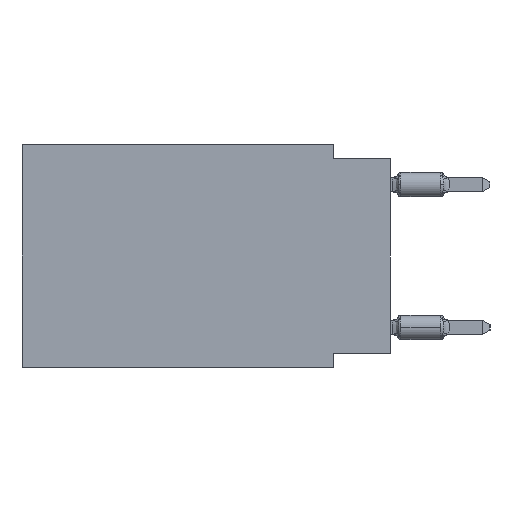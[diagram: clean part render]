
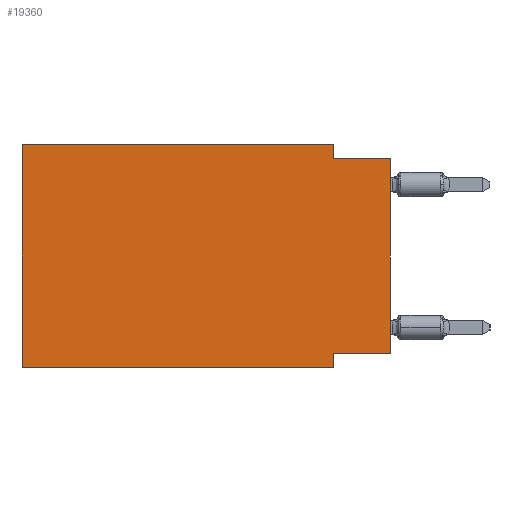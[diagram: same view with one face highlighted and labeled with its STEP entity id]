
A CAD part, left-side view. The second image highlights one B-rep face of the part: STEP entity #19360.
In plain terms, the highlighted planar face has unit normal (-1, 0, 0).
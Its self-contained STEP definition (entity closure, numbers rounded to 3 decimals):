
#542 = VERTEX_POINT ( 'NONE', #7815 ) ;
#738 = FACE_OUTER_BOUND ( 'NONE', #15789, .T. ) ;
#1135 = CARTESIAN_POINT ( 'NONE',  ( 0., 16.383, 0. ) ) ;
#1279 = VECTOR ( 'NONE', #3254, 1000. ) ;
#2408 = VECTOR ( 'NONE', #6625, 1000. ) ;
#2459 = PLANE ( 'NONE',  #6780 ) ;
#2726 = DIRECTION ( 'NONE',  ( 0., -1., 0. ) ) ;
#2769 = VERTEX_POINT ( 'NONE', #12628 ) ;
#2966 = VECTOR ( 'NONE', #13197, 1000. ) ;
#3254 = DIRECTION ( 'NONE',  ( 0., 0., -1. ) ) ;
#3585 = VECTOR ( 'NONE', #21722, 1000. ) ;
#3939 = CARTESIAN_POINT ( 'NONE',  ( 0., 2.54, -9.271 ) ) ;
#4304 = VECTOR ( 'NONE', #8159, 1000. ) ;
#4620 = LINE ( 'NONE', #17834, #4304 ) ;
#4680 = LINE ( 'NONE', #23396, #2408 ) ;
#4748 = VECTOR ( 'NONE', #19004, 1000. ) ;
#5095 = CARTESIAN_POINT ( 'NONE',  ( 0., 16.383, -9.906 ) ) ;
#5386 = VERTEX_POINT ( 'NONE', #3939 ) ;
#5447 = CARTESIAN_POINT ( 'NONE',  ( 0., 0., -9.271 ) ) ;
#5783 = ORIENTED_EDGE ( 'NONE', *, *, #18424, .F. ) ;
#6580 = VERTEX_POINT ( 'NONE', #20366 ) ;
#6625 = DIRECTION ( 'NONE',  ( 0., -1., 0. ) ) ;
#6780 = AXIS2_PLACEMENT_3D ( 'NONE', #13448, #23104, #19213 ) ;
#7251 = VERTEX_POINT ( 'NONE', #5095 ) ;
#7281 = EDGE_CURVE ( 'NONE', #7251, #22272, #20169, .T. ) ;
#7815 = CARTESIAN_POINT ( 'NONE',  ( 0., 0., -0.635 ) ) ;
#7839 = VERTEX_POINT ( 'NONE', #13263 ) ;
#8159 = DIRECTION ( 'NONE',  ( 0., -1., 0. ) ) ;
#8427 = EDGE_CURVE ( 'NONE', #5386, #7839, #16635, .T. ) ;
#10823 = LINE ( 'NONE', #5447, #3585 ) ;
#10858 = ORIENTED_EDGE ( 'NONE', *, *, #13894, .F. ) ;
#11376 = ORIENTED_EDGE ( 'NONE', *, *, #7281, .F. ) ;
#11389 = LINE ( 'NONE', #22779, #4748 ) ;
#11809 = EDGE_CURVE ( 'NONE', #7251, #7839, #4680, .T. ) ;
#12370 = LINE ( 'NONE', #1135, #22649 ) ;
#12628 = CARTESIAN_POINT ( 'NONE',  ( 0., 2.54, 0. ) ) ;
#12911 = EDGE_CURVE ( 'NONE', #22272, #2769, #12370, .T. ) ;
#13197 = DIRECTION ( 'NONE',  ( 0., 0., -1. ) ) ;
#13263 = CARTESIAN_POINT ( 'NONE',  ( 0., 2.54, -9.906 ) ) ;
#13448 = CARTESIAN_POINT ( 'NONE',  ( 0., 16.383, 0. ) ) ;
#13894 = EDGE_CURVE ( 'NONE', #6580, #542, #4620, .T. ) ;
#14370 = CARTESIAN_POINT ( 'NONE',  ( 0., 2.54, 0. ) ) ;
#15590 = EDGE_CURVE ( 'NONE', #22223, #5386, #10823, .T. ) ;
#15740 = CARTESIAN_POINT ( 'NONE',  ( 0., 0., -9.271 ) ) ;
#15789 = EDGE_LOOP ( 'NONE', ( #21813, #10858, #5783, #22189, #11376, #16854, #18591, #17774 ) ) ;
#16044 = EDGE_CURVE ( 'NONE', #22223, #542, #11389, .T. ) ;
#16635 = LINE ( 'NONE', #24098, #2966 ) ;
#16854 = ORIENTED_EDGE ( 'NONE', *, *, #11809, .T. ) ;
#17774 = ORIENTED_EDGE ( 'NONE', *, *, #15590, .F. ) ;
#17834 = CARTESIAN_POINT ( 'NONE',  ( 0., 0., -0.635 ) ) ;
#18325 = CARTESIAN_POINT ( 'NONE',  ( 0., 16.383, 0. ) ) ;
#18424 = EDGE_CURVE ( 'NONE', #2769, #6580, #20014, .T. ) ;
#18591 = ORIENTED_EDGE ( 'NONE', *, *, #8427, .F. ) ;
#19004 = DIRECTION ( 'NONE',  ( 0., 0., 1. ) ) ;
#19213 = DIRECTION ( 'NONE',  ( 0., 0., -1. ) ) ;
#19360 = ADVANCED_FACE ( 'NONE', ( #738 ), #2459, .F. ) ;
#19538 = CARTESIAN_POINT ( 'NONE',  ( 0., 16.383, 0. ) ) ;
#20014 = LINE ( 'NONE', #14370, #1279 ) ;
#20169 = LINE ( 'NONE', #18325, #22438 ) ;
#20366 = CARTESIAN_POINT ( 'NONE',  ( 0., 2.54, -0.635 ) ) ;
#21722 = DIRECTION ( 'NONE',  ( 0., 1., 0. ) ) ;
#21813 = ORIENTED_EDGE ( 'NONE', *, *, #16044, .T. ) ;
#22189 = ORIENTED_EDGE ( 'NONE', *, *, #12911, .F. ) ;
#22223 = VERTEX_POINT ( 'NONE', #15740 ) ;
#22272 = VERTEX_POINT ( 'NONE', #19538 ) ;
#22438 = VECTOR ( 'NONE', #23819, 1000. ) ;
#22649 = VECTOR ( 'NONE', #2726, 1000. ) ;
#22779 = CARTESIAN_POINT ( 'NONE',  ( 0., 0., 0. ) ) ;
#23104 = DIRECTION ( 'NONE',  ( 1., 0., 0. ) ) ;
#23396 = CARTESIAN_POINT ( 'NONE',  ( 0., 16.383, -9.906 ) ) ;
#23819 = DIRECTION ( 'NONE',  ( 0., 0., 1. ) ) ;
#24098 = CARTESIAN_POINT ( 'NONE',  ( 0., 2.54, -9.906 ) ) ;
